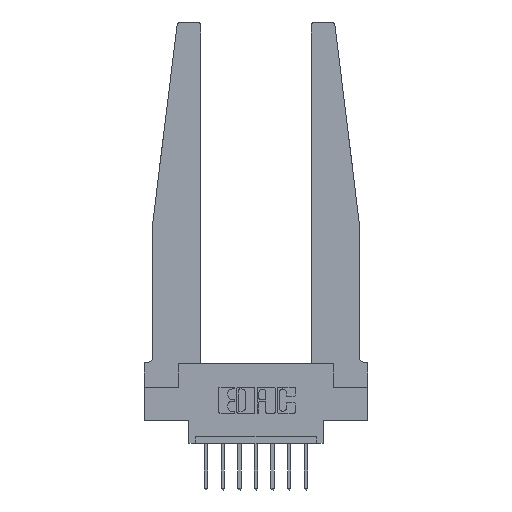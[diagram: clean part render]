
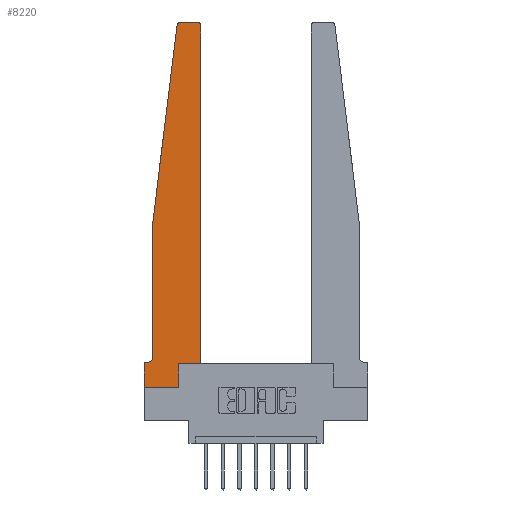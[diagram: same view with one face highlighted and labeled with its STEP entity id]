
A CAD part, top view. The second image highlights one B-rep face of the part: STEP entity #8220.
In plain terms, the highlighted planar face has unit normal (0, 0, 1).
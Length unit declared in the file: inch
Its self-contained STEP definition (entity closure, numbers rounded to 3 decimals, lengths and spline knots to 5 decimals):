
#4 = VECTOR ( 'NONE', #12723, 39.37008 ) ;
#917 = CARTESIAN_POINT ( 'NONE',  ( 0., 0.1875, 0.37 ) ) ;
#1265 = AXIS2_PLACEMENT_3D ( 'NONE', #8052, #1442, #11147 ) ;
#1271 = LINE ( 'NONE', #12559, #4019 ) ;
#1442 = DIRECTION ( 'NONE',  ( 0., 0., 1. ) ) ;
#1452 = EDGE_CURVE ( 'NONE', #9046, #12142, #3805, .T. ) ;
#1534 = CARTESIAN_POINT ( 'NONE',  ( 0.015, 0.2375, 0.37 ) ) ;
#1676 = VERTEX_POINT ( 'NONE', #6570 ) ;
#2010 = EDGE_CURVE ( 'NONE', #1676, #6747, #13957, .T. ) ;
#2025 = CARTESIAN_POINT ( 'NONE',  ( 0., 0., 0.37 ) ) ;
#2399 = VECTOR ( 'NONE', #7630, 39.37008 ) ;
#2576 = CARTESIAN_POINT ( 'NONE',  ( 0.2605, 0.18, 0.37 ) ) ;
#2836 = DIRECTION ( 'NONE',  ( -1., 0., 0. ) ) ;
#3272 = EDGE_CURVE ( 'NONE', #10701, #4504, #6000, .T. ) ;
#3632 = CARTESIAN_POINT ( 'NONE',  ( 0.24675, 2.72367, 0.37 ) ) ;
#3805 = LINE ( 'NONE', #8368, #14405 ) ;
#3864 = CARTESIAN_POINT ( 'NONE',  ( 0.395, 2.75, 0.37 ) ) ;
#3900 = DIRECTION ( 'NONE',  ( 1., 0., 0. ) ) ;
#4019 = VECTOR ( 'NONE', #5779, 39.37008 ) ;
#4085 = ORIENTED_EDGE ( 'NONE', *, *, #8704, .T. ) ;
#4169 = DIRECTION ( 'NONE',  ( 0., 0., 1. ) ) ;
#4236 = VECTOR ( 'NONE', #3900, 39.37008 ) ;
#4504 = VERTEX_POINT ( 'NONE', #11325 ) ;
#4543 = VECTOR ( 'NONE', #13292, 39.37008 ) ;
#4712 = FACE_OUTER_BOUND ( 'NONE', #5808, .T. ) ;
#4765 = CARTESIAN_POINT ( 'NONE',  ( 0.065, 1.25, 0.37 ) ) ;
#5228 = DIRECTION ( 'NONE',  ( 0., -1., 0. ) ) ;
#5666 = LINE ( 'NONE', #13378, #9558 ) ;
#5761 = EDGE_CURVE ( 'NONE', #12142, #10701, #13100, .T. ) ;
#5779 = DIRECTION ( 'NONE',  ( 1., 0., 0. ) ) ;
#5808 = EDGE_LOOP ( 'NONE', ( #7827, #11738, #4085, #11527, #12734, #8275, #9539, #13098, #13978, #13314, #9185, #6521 ) ) ;
#6000 = LINE ( 'NONE', #12852, #4236 ) ;
#6413 = DIRECTION ( 'NONE',  ( 1., 0., 0. ) ) ;
#6521 = ORIENTED_EDGE ( 'NONE', *, *, #2010, .T. ) ;
#6570 = CARTESIAN_POINT ( 'NONE',  ( 0.425, 2.72, 0.37 ) ) ;
#6747 = VERTEX_POINT ( 'NONE', #3864 ) ;
#6819 = LINE ( 'NONE', #4765, #4543 ) ;
#7116 = CARTESIAN_POINT ( 'NONE',  ( 0., 0., 0.37 ) ) ;
#7298 = DIRECTION ( 'NONE',  ( 1., 0., 0. ) ) ;
#7574 = VERTEX_POINT ( 'NONE', #2576 ) ;
#7630 = DIRECTION ( 'NONE',  ( 0., 1., 0. ) ) ;
#7695 = DIRECTION ( 'NONE',  ( 0., 0., 1. ) ) ;
#7827 = ORIENTED_EDGE ( 'NONE', *, *, #13690, .T. ) ;
#8052 = CARTESIAN_POINT ( 'NONE',  ( 0., 0.1875, 0.37 ) ) ;
#8220 = ADVANCED_FACE ( 'NONE', ( #4712 ), #13670, .T. ) ;
#8225 = DIRECTION ( 'NONE',  ( 0., 0., -1. ) ) ;
#8275 = ORIENTED_EDGE ( 'NONE', *, *, #1452, .T. ) ;
#8293 = DIRECTION ( 'NONE',  ( -1., 0., 0. ) ) ;
#8368 = CARTESIAN_POINT ( 'NONE',  ( 0.065, 0.1875, 0.37 ) ) ;
#8482 = CIRCLE ( 'NONE', #9654, 0.03 ) ;
#8704 = EDGE_CURVE ( 'NONE', #10217, #12180, #6819, .T. ) ;
#8727 = VECTOR ( 'NONE', #5228, 39.37008 ) ;
#9046 = VERTEX_POINT ( 'NONE', #9934 ) ;
#9185 = ORIENTED_EDGE ( 'NONE', *, *, #12964, .T. ) ;
#9539 = ORIENTED_EDGE ( 'NONE', *, *, #5761, .T. ) ;
#9553 = CARTESIAN_POINT ( 'NONE',  ( 0.395, 2.72, 0.37 ) ) ;
#9558 = VECTOR ( 'NONE', #11286, 39.37008 ) ;
#9584 = LINE ( 'NONE', #10544, #4 ) ;
#9654 = AXIS2_PLACEMENT_3D ( 'NONE', #10783, #7695, #6413 ) ;
#9934 = CARTESIAN_POINT ( 'NONE',  ( 0.015, 0.1875, 0.37 ) ) ;
#9995 = CARTESIAN_POINT ( 'NONE',  ( 0.065, 0.2375, 0.37 ) ) ;
#10173 = CARTESIAN_POINT ( 'NONE',  ( 0.065, 1.25, 0.37 ) ) ;
#10217 = VERTEX_POINT ( 'NONE', #3632 ) ;
#10479 = EDGE_CURVE ( 'NONE', #4504, #7574, #10855, .T. ) ;
#10544 = CARTESIAN_POINT ( 'NONE',  ( 0.065, 1.25, 0.37 ) ) ;
#10672 = EDGE_CURVE ( 'NONE', #12180, #11463, #9584, .T. ) ;
#10701 = VERTEX_POINT ( 'NONE', #7116 ) ;
#10783 = CARTESIAN_POINT ( 'NONE',  ( 0.27653, 2.72, 0.37 ) ) ;
#10855 = LINE ( 'NONE', #14185, #2399 ) ;
#11147 = DIRECTION ( 'NONE',  ( 1., 0., 0. ) ) ;
#11191 = AXIS2_PLACEMENT_3D ( 'NONE', #9553, #4169, #7298 ) ;
#11286 = DIRECTION ( 'NONE',  ( -1., 0., 0. ) ) ;
#11301 = CARTESIAN_POINT ( 'NONE',  ( 0.425, 0.18, 0.37 ) ) ;
#11325 = CARTESIAN_POINT ( 'NONE',  ( 0.2605, 0., 0.37 ) ) ;
#11463 = VERTEX_POINT ( 'NONE', #9995 ) ;
#11495 = VECTOR ( 'NONE', #13392, 39.37008 ) ;
#11527 = ORIENTED_EDGE ( 'NONE', *, *, #10672, .T. ) ;
#11658 = EDGE_CURVE ( 'NONE', #11463, #9046, #12173, .T. ) ;
#11738 = ORIENTED_EDGE ( 'NONE', *, *, #13622, .T. ) ;
#12142 = VERTEX_POINT ( 'NONE', #917 ) ;
#12173 = CIRCLE ( 'NONE', #12400, 0.05 ) ;
#12180 = VERTEX_POINT ( 'NONE', #10173 ) ;
#12198 = EDGE_CURVE ( 'NONE', #7574, #13149, #1271, .T. ) ;
#12385 = VERTEX_POINT ( 'NONE', #12844 ) ;
#12400 = AXIS2_PLACEMENT_3D ( 'NONE', #1534, #8225, #8293 ) ;
#12559 = CARTESIAN_POINT ( 'NONE',  ( 0.425, 0.18, 0.37 ) ) ;
#12723 = DIRECTION ( 'NONE',  ( 0., -1., 0. ) ) ;
#12734 = ORIENTED_EDGE ( 'NONE', *, *, #11658, .T. ) ;
#12742 = CARTESIAN_POINT ( 'NONE',  ( 0.425, 0.18, 0.37 ) ) ;
#12844 = CARTESIAN_POINT ( 'NONE',  ( 0.27653, 2.75, 0.37 ) ) ;
#12852 = CARTESIAN_POINT ( 'NONE',  ( 0., 0., 0.37 ) ) ;
#12964 = EDGE_CURVE ( 'NONE', #13149, #1676, #13463, .T. ) ;
#13098 = ORIENTED_EDGE ( 'NONE', *, *, #3272, .T. ) ;
#13100 = LINE ( 'NONE', #2025, #8727 ) ;
#13149 = VERTEX_POINT ( 'NONE', #12742 ) ;
#13292 = DIRECTION ( 'NONE',  ( -0.122, -0.992, 0. ) ) ;
#13314 = ORIENTED_EDGE ( 'NONE', *, *, #12198, .T. ) ;
#13378 = CARTESIAN_POINT ( 'NONE',  ( 0.25, 2.75, 0.37 ) ) ;
#13392 = DIRECTION ( 'NONE',  ( 0., 1., 0. ) ) ;
#13463 = LINE ( 'NONE', #11301, #11495 ) ;
#13622 = EDGE_CURVE ( 'NONE', #12385, #10217, #8482, .T. ) ;
#13670 = PLANE ( 'NONE',  #1265 ) ;
#13690 = EDGE_CURVE ( 'NONE', #6747, #12385, #5666, .T. ) ;
#13957 = CIRCLE ( 'NONE', #11191, 0.03 ) ;
#13978 = ORIENTED_EDGE ( 'NONE', *, *, #10479, .T. ) ;
#14185 = CARTESIAN_POINT ( 'NONE',  ( 0.2605, 0.18, 0.37 ) ) ;
#14405 = VECTOR ( 'NONE', #2836, 39.37008 ) ;
